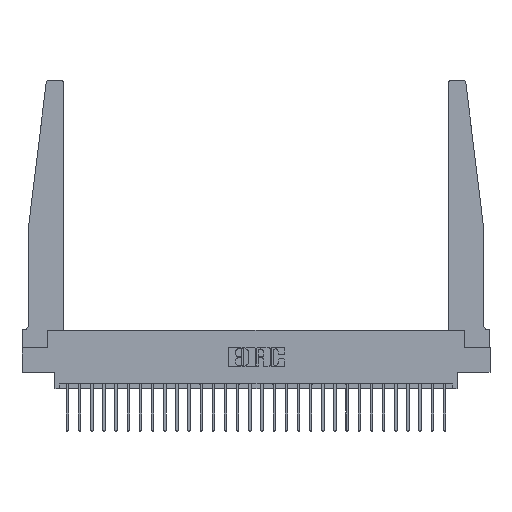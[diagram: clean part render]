
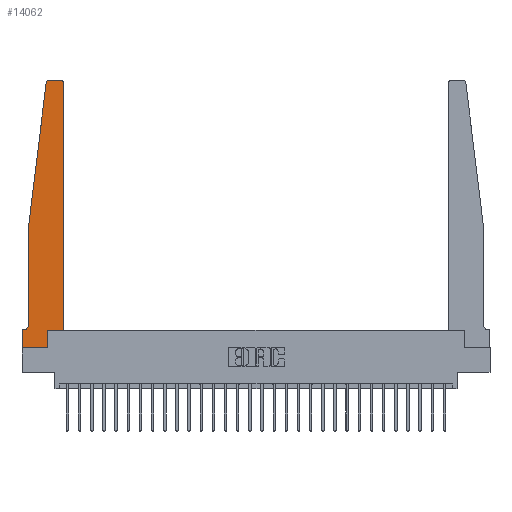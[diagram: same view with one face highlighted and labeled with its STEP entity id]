
A CAD part, top view. The second image highlights one B-rep face of the part: STEP entity #14062.
In plain terms, the highlighted planar face has unit normal (0, 0, 1).
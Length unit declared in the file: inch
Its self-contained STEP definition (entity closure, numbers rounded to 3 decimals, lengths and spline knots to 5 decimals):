
#299 = CARTESIAN_POINT ( 'NONE',  ( 0.065, 0.1875, 0.37 ) ) ;
#517 = LINE ( 'NONE', #3707, #21531 ) ;
#522 = AXIS2_PLACEMENT_3D ( 'NONE', #8252, #23014, #10400 ) ;
#858 = CARTESIAN_POINT ( 'NONE',  ( 0.425, 0.18, 0.37 ) ) ;
#948 = CIRCLE ( 'NONE', #18266, 0.03 ) ;
#1118 = ORIENTED_EDGE ( 'NONE', *, *, #25400, .T. ) ;
#1304 = DIRECTION ( 'NONE',  ( 0., 0., 1. ) ) ;
#1760 = CARTESIAN_POINT ( 'NONE',  ( 0.27653, 2.75, 0.37 ) ) ;
#2640 = ORIENTED_EDGE ( 'NONE', *, *, #27106, .T. ) ;
#3707 = CARTESIAN_POINT ( 'NONE',  ( 0., 0., 0.37 ) ) ;
#3855 = VERTEX_POINT ( 'NONE', #1760 ) ;
#4258 = ORIENTED_EDGE ( 'NONE', *, *, #20515, .T. ) ;
#4476 = LINE ( 'NONE', #16786, #9385 ) ;
#4552 = EDGE_CURVE ( 'NONE', #6047, #9477, #16185, .T. ) ;
#5112 = CARTESIAN_POINT ( 'NONE',  ( 0.25, 2.75, 0.37 ) ) ;
#5134 = CIRCLE ( 'NONE', #522, 0.03 ) ;
#5647 = EDGE_CURVE ( 'NONE', #11519, #3855, #19728, .T. ) ;
#5771 = VERTEX_POINT ( 'NONE', #20305 ) ;
#6047 = VERTEX_POINT ( 'NONE', #10617 ) ;
#6122 = ORIENTED_EDGE ( 'NONE', *, *, #25364, .T. ) ;
#6940 = VECTOR ( 'NONE', #26112, 39.37008 ) ;
#7234 = DIRECTION ( 'NONE',  ( -0.122, -0.992, 0. ) ) ;
#7235 = VERTEX_POINT ( 'NONE', #858 ) ;
#7317 = ORIENTED_EDGE ( 'NONE', *, *, #24497, .T. ) ;
#7554 = DIRECTION ( 'NONE',  ( 0., 0., 1. ) ) ;
#7723 = CARTESIAN_POINT ( 'NONE',  ( 0.2605, 0.18, 0.37 ) ) ;
#7837 = VERTEX_POINT ( 'NONE', #21486 ) ;
#8066 = DIRECTION ( 'NONE',  ( 0., 0., -1. ) ) ;
#8252 = CARTESIAN_POINT ( 'NONE',  ( 0.395, 2.72, 0.37 ) ) ;
#8532 = DIRECTION ( 'NONE',  ( 1., 0., 0. ) ) ;
#8845 = VERTEX_POINT ( 'NONE', #16098 ) ;
#8973 = FACE_OUTER_BOUND ( 'NONE', #24648, .T. ) ;
#9385 = VECTOR ( 'NONE', #12554, 39.37008 ) ;
#9437 = LINE ( 'NONE', #299, #25582 ) ;
#9477 = VERTEX_POINT ( 'NONE', #26799 ) ;
#10400 = DIRECTION ( 'NONE',  ( 1., 0., 0. ) ) ;
#10617 = CARTESIAN_POINT ( 'NONE',  ( 0.065, 0.2375, 0.37 ) ) ;
#10622 = CARTESIAN_POINT ( 'NONE',  ( 0.065, 1.25, 0.37 ) ) ;
#10861 = CARTESIAN_POINT ( 'NONE',  ( 0.2605, 0.18, 0.37 ) ) ;
#10877 = ORIENTED_EDGE ( 'NONE', *, *, #11581, .T. ) ;
#11337 = ORIENTED_EDGE ( 'NONE', *, *, #14351, .T. ) ;
#11510 = CARTESIAN_POINT ( 'NONE',  ( 0.065, 1.25, 0.37 ) ) ;
#11519 = VERTEX_POINT ( 'NONE', #24168 ) ;
#11581 = EDGE_CURVE ( 'NONE', #3855, #5771, #948, .T. ) ;
#11945 = LINE ( 'NONE', #11510, #6940 ) ;
#12554 = DIRECTION ( 'NONE',  ( 0., -1., 0. ) ) ;
#12675 = EDGE_CURVE ( 'NONE', #5771, #26803, #18989, .T. ) ;
#12965 = VECTOR ( 'NONE', #23499, 39.37008 ) ;
#13066 = VERTEX_POINT ( 'NONE', #10861 ) ;
#13241 = ORIENTED_EDGE ( 'NONE', *, *, #12675, .T. ) ;
#13393 = VECTOR ( 'NONE', #7234, 39.37008 ) ;
#13488 = VECTOR ( 'NONE', #21979, 39.37008 ) ;
#13634 = LINE ( 'NONE', #19374, #12965 ) ;
#14062 = ADVANCED_FACE ( 'NONE', ( #8973 ), #26430, .T. ) ;
#14274 = CARTESIAN_POINT ( 'NONE',  ( 0.425, 2.72, 0.37 ) ) ;
#14351 = EDGE_CURVE ( 'NONE', #7235, #15235, #13634, .T. ) ;
#14569 = AXIS2_PLACEMENT_3D ( 'NONE', #20120, #1304, #15993 ) ;
#14631 = ORIENTED_EDGE ( 'NONE', *, *, #18488, .T. ) ;
#14773 = EDGE_CURVE ( 'NONE', #13066, #7235, #22164, .T. ) ;
#15235 = VERTEX_POINT ( 'NONE', #14274 ) ;
#15695 = ORIENTED_EDGE ( 'NONE', *, *, #14773, .T. ) ;
#15993 = DIRECTION ( 'NONE',  ( 1., 0., 0. ) ) ;
#16098 = CARTESIAN_POINT ( 'NONE',  ( 0., 0., 0.37 ) ) ;
#16185 = CIRCLE ( 'NONE', #24096, 0.05 ) ;
#16262 = DIRECTION ( 'NONE',  ( 0., 1., 0. ) ) ;
#16333 = ORIENTED_EDGE ( 'NONE', *, *, #5647, .T. ) ;
#16786 = CARTESIAN_POINT ( 'NONE',  ( 0., 0., 0.37 ) ) ;
#17092 = DIRECTION ( 'NONE',  ( -1., 0., 0. ) ) ;
#18266 = AXIS2_PLACEMENT_3D ( 'NONE', #20217, #7554, #22338 ) ;
#18488 = EDGE_CURVE ( 'NONE', #7837, #13066, #25468, .T. ) ;
#18989 = LINE ( 'NONE', #22016, #13393 ) ;
#19084 = CARTESIAN_POINT ( 'NONE',  ( 0.425, 0.18, 0.37 ) ) ;
#19251 = VECTOR ( 'NONE', #16262, 39.37008 ) ;
#19374 = CARTESIAN_POINT ( 'NONE',  ( 0.425, 0.18, 0.37 ) ) ;
#19728 = LINE ( 'NONE', #5112, #13488 ) ;
#20120 = CARTESIAN_POINT ( 'NONE',  ( 0., 0.1875, 0.37 ) ) ;
#20217 = CARTESIAN_POINT ( 'NONE',  ( 0.27653, 2.72, 0.37 ) ) ;
#20305 = CARTESIAN_POINT ( 'NONE',  ( 0.24675, 2.72367, 0.37 ) ) ;
#20515 = EDGE_CURVE ( 'NONE', #26803, #6047, #11945, .T. ) ;
#20545 = DIRECTION ( 'NONE',  ( 1., 0., 0. ) ) ;
#20730 = CARTESIAN_POINT ( 'NONE',  ( 0.015, 0.2375, 0.37 ) ) ;
#21034 = CARTESIAN_POINT ( 'NONE',  ( 0., 0.1875, 0.37 ) ) ;
#21486 = CARTESIAN_POINT ( 'NONE',  ( 0.2605, 0., 0.37 ) ) ;
#21531 = VECTOR ( 'NONE', #20545, 39.37008 ) ;
#21979 = DIRECTION ( 'NONE',  ( -1., 0., 0. ) ) ;
#22016 = CARTESIAN_POINT ( 'NONE',  ( 0.065, 1.25, 0.37 ) ) ;
#22164 = LINE ( 'NONE', #19084, #27060 ) ;
#22338 = DIRECTION ( 'NONE',  ( 1., 0., 0. ) ) ;
#22589 = VERTEX_POINT ( 'NONE', #21034 ) ;
#22829 = DIRECTION ( 'NONE',  ( -1., 0., 0. ) ) ;
#23014 = DIRECTION ( 'NONE',  ( 0., 0., 1. ) ) ;
#23499 = DIRECTION ( 'NONE',  ( 0., 1., 0. ) ) ;
#24096 = AXIS2_PLACEMENT_3D ( 'NONE', #20730, #8066, #22829 ) ;
#24168 = CARTESIAN_POINT ( 'NONE',  ( 0.395, 2.75, 0.37 ) ) ;
#24497 = EDGE_CURVE ( 'NONE', #9477, #22589, #9437, .T. ) ;
#24648 = EDGE_LOOP ( 'NONE', ( #16333, #10877, #13241, #4258, #27121, #7317, #1118, #2640, #14631, #15695, #11337, #6122 ) ) ;
#25364 = EDGE_CURVE ( 'NONE', #15235, #11519, #5134, .T. ) ;
#25400 = EDGE_CURVE ( 'NONE', #22589, #8845, #4476, .T. ) ;
#25468 = LINE ( 'NONE', #7723, #19251 ) ;
#25582 = VECTOR ( 'NONE', #17092, 39.37008 ) ;
#26112 = DIRECTION ( 'NONE',  ( 0., -1., 0. ) ) ;
#26430 = PLANE ( 'NONE',  #14569 ) ;
#26799 = CARTESIAN_POINT ( 'NONE',  ( 0.015, 0.1875, 0.37 ) ) ;
#26803 = VERTEX_POINT ( 'NONE', #10622 ) ;
#27060 = VECTOR ( 'NONE', #8532, 39.37008 ) ;
#27106 = EDGE_CURVE ( 'NONE', #8845, #7837, #517, .T. ) ;
#27121 = ORIENTED_EDGE ( 'NONE', *, *, #4552, .T. ) ;
